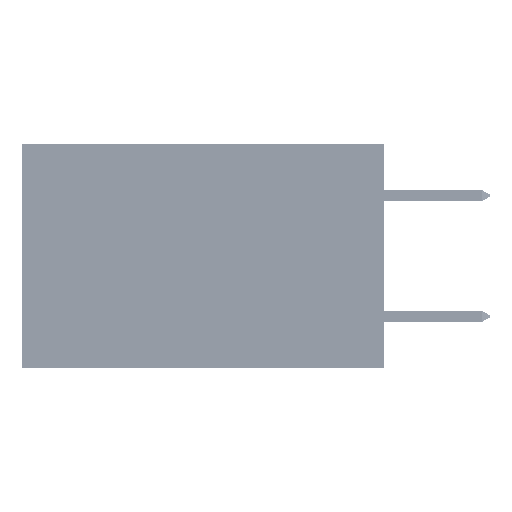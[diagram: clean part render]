
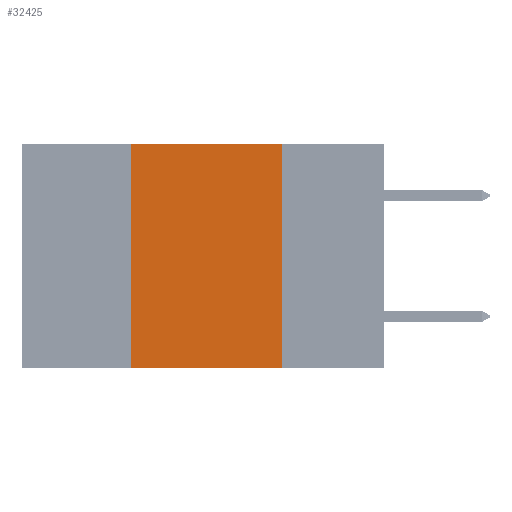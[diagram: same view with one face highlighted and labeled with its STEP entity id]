
A CAD part, left-side view. The second image highlights one B-rep face of the part: STEP entity #32425.
In plain terms, the highlighted planar face has unit normal (-1, 0, 0).
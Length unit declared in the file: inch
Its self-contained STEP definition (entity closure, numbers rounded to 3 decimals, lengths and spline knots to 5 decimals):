
#241 = FACE_OUTER_BOUND ( 'NONE', #37810, .T. ) ;
#568 = EDGE_CURVE ( 'NONE', #43495, #3155, #28917, .T. ) ;
#1236 = VECTOR ( 'NONE', #18280, 39.37008 ) ;
#1889 = LINE ( 'NONE', #29827, #1236 ) ;
#2543 = VECTOR ( 'NONE', #15799, 39.37008 ) ;
#2974 = DIRECTION ( 'NONE',  ( 1., 0., 0. ) ) ;
#3155 = VERTEX_POINT ( 'NONE', #27648 ) ;
#3247 = VECTOR ( 'NONE', #30152, 39.37008 ) ;
#5863 = CARTESIAN_POINT ( 'NONE',  ( 0., 0.17, 0. ) ) ;
#8147 = EDGE_CURVE ( 'NONE', #32814, #3155, #16500, .T. ) ;
#10190 = DIRECTION ( 'NONE',  ( 0., 0., -1. ) ) ;
#11271 = CARTESIAN_POINT ( 'NONE',  ( 0., 0.17, 0. ) ) ;
#11977 = CARTESIAN_POINT ( 'NONE',  ( 0., 0.42, 0. ) ) ;
#15799 = DIRECTION ( 'NONE',  ( 0., -1., 0. ) ) ;
#16091 = AXIS2_PLACEMENT_3D ( 'NONE', #42480, #2974, #10190 ) ;
#16500 = LINE ( 'NONE', #11271, #31532 ) ;
#18280 = DIRECTION ( 'NONE',  ( 0., 0., 1. ) ) ;
#25287 = EDGE_CURVE ( 'NONE', #52016, #32814, #37730, .T. ) ;
#27648 = CARTESIAN_POINT ( 'NONE',  ( 0., 0.17, -0.37 ) ) ;
#28917 = LINE ( 'NONE', #31043, #2543 ) ;
#29356 = EDGE_CURVE ( 'NONE', #43495, #52016, #1889, .T. ) ;
#29827 = CARTESIAN_POINT ( 'NONE',  ( 0., 0.42, 0. ) ) ;
#30152 = DIRECTION ( 'NONE',  ( 0., -1., 0. ) ) ;
#31043 = CARTESIAN_POINT ( 'NONE',  ( 0., 0.6, -0.37 ) ) ;
#31532 = VECTOR ( 'NONE', #39310, 39.37008 ) ;
#32425 = ADVANCED_FACE ( 'NONE', ( #241 ), #47064, .F. ) ;
#32814 = VERTEX_POINT ( 'NONE', #5863 ) ;
#37730 = LINE ( 'NONE', #45834, #3247 ) ;
#37810 = EDGE_LOOP ( 'NONE', ( #41570, #50198, #42489, #40761 ) ) ;
#39310 = DIRECTION ( 'NONE',  ( 0., 0., -1. ) ) ;
#40761 = ORIENTED_EDGE ( 'NONE', *, *, #568, .T. ) ;
#41570 = ORIENTED_EDGE ( 'NONE', *, *, #8147, .F. ) ;
#42480 = CARTESIAN_POINT ( 'NONE',  ( 0., 0.6, 0. ) ) ;
#42489 = ORIENTED_EDGE ( 'NONE', *, *, #29356, .F. ) ;
#43495 = VERTEX_POINT ( 'NONE', #50148 ) ;
#45834 = CARTESIAN_POINT ( 'NONE',  ( 0., 0.6, 0. ) ) ;
#47064 = PLANE ( 'NONE',  #16091 ) ;
#50148 = CARTESIAN_POINT ( 'NONE',  ( 0., 0.42, -0.37 ) ) ;
#50198 = ORIENTED_EDGE ( 'NONE', *, *, #25287, .F. ) ;
#52016 = VERTEX_POINT ( 'NONE', #11977 ) ;
